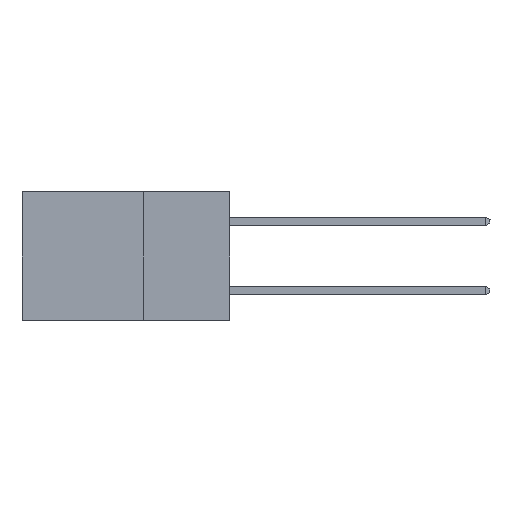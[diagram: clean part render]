
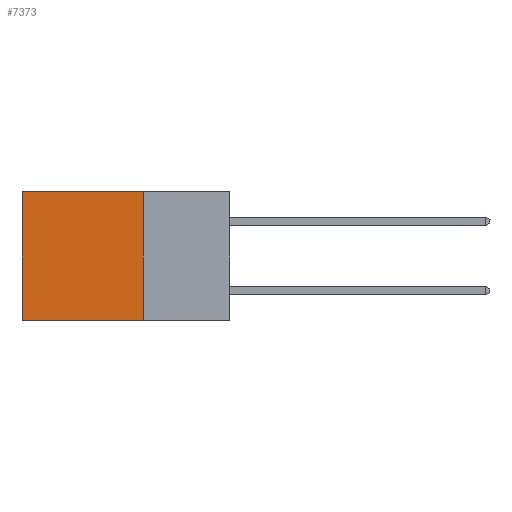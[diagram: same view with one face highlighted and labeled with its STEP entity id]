
A CAD part, left-side view. The second image highlights one B-rep face of the part: STEP entity #7373.
In plain terms, the highlighted planar face has unit normal (-1, 0, 0).
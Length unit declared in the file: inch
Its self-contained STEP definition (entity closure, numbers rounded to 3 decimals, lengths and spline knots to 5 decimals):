
#204 = VERTEX_POINT ( 'NONE', #3037 ) ;
#454 = EDGE_CURVE ( 'NONE', #10063, #702, #16908, .T. ) ;
#702 = VERTEX_POINT ( 'NONE', #12902 ) ;
#1126 = AXIS2_PLACEMENT_3D ( 'NONE', #7693, #13541, #2274 ) ;
#1356 = DIRECTION ( 'NONE',  ( 0., 1., 0. ) ) ;
#1970 = VECTOR ( 'NONE', #1356, 39.37008 ) ;
#2274 = DIRECTION ( 'NONE',  ( 0., 0., -1. ) ) ;
#2349 = LINE ( 'NONE', #17749, #11010 ) ;
#2656 = DIRECTION ( 'NONE',  ( 0., 0., -1. ) ) ;
#3037 = CARTESIAN_POINT ( 'NONE',  ( 0.2615, 0.6, -0.37 ) ) ;
#4178 = CARTESIAN_POINT ( 'NONE',  ( 0.2615, 0.25, -0.37 ) ) ;
#4546 = ORIENTED_EDGE ( 'NONE', *, *, #6266, .F. ) ;
#4577 = CARTESIAN_POINT ( 'NONE',  ( 0.2615, 0.25, -0.37 ) ) ;
#4629 = VECTOR ( 'NONE', #11249, 39.37008 ) ;
#4939 = ORIENTED_EDGE ( 'NONE', *, *, #10504, .T. ) ;
#6266 = EDGE_CURVE ( 'NONE', #702, #204, #16420, .T. ) ;
#6794 = CARTESIAN_POINT ( 'NONE',  ( 0.2615, 0.25, 0. ) ) ;
#6816 = EDGE_LOOP ( 'NONE', ( #16819, #4546, #14680, #4939 ) ) ;
#7373 = ADVANCED_FACE ( 'NONE', ( #14811 ), #14894, .F. ) ;
#7693 = CARTESIAN_POINT ( 'NONE',  ( 0.2615, 0.25, -0.37 ) ) ;
#7930 = CARTESIAN_POINT ( 'NONE',  ( 0.2615, 0.6, 0. ) ) ;
#8040 = VERTEX_POINT ( 'NONE', #7930 ) ;
#8641 = LINE ( 'NONE', #12512, #4629 ) ;
#9120 = DIRECTION ( 'NONE',  ( 0., 1., 0. ) ) ;
#10063 = VERTEX_POINT ( 'NONE', #6794 ) ;
#10504 = EDGE_CURVE ( 'NONE', #10063, #8040, #2349, .T. ) ;
#10515 = VECTOR ( 'NONE', #2656, 39.37008 ) ;
#11010 = VECTOR ( 'NONE', #9120, 39.37008 ) ;
#11249 = DIRECTION ( 'NONE',  ( 0., 0., -1. ) ) ;
#12512 = CARTESIAN_POINT ( 'NONE',  ( 0.2615, 0.6, -0.37 ) ) ;
#12902 = CARTESIAN_POINT ( 'NONE',  ( 0.2615, 0.25, -0.37 ) ) ;
#13541 = DIRECTION ( 'NONE',  ( 1., 0., 0. ) ) ;
#14680 = ORIENTED_EDGE ( 'NONE', *, *, #454, .F. ) ;
#14811 = FACE_OUTER_BOUND ( 'NONE', #6816, .T. ) ;
#14894 = PLANE ( 'NONE',  #1126 ) ;
#16420 = LINE ( 'NONE', #4178, #1970 ) ;
#16464 = EDGE_CURVE ( 'NONE', #8040, #204, #8641, .T. ) ;
#16819 = ORIENTED_EDGE ( 'NONE', *, *, #16464, .T. ) ;
#16908 = LINE ( 'NONE', #4577, #10515 ) ;
#17749 = CARTESIAN_POINT ( 'NONE',  ( 0.2615, 0.25, 0. ) ) ;
